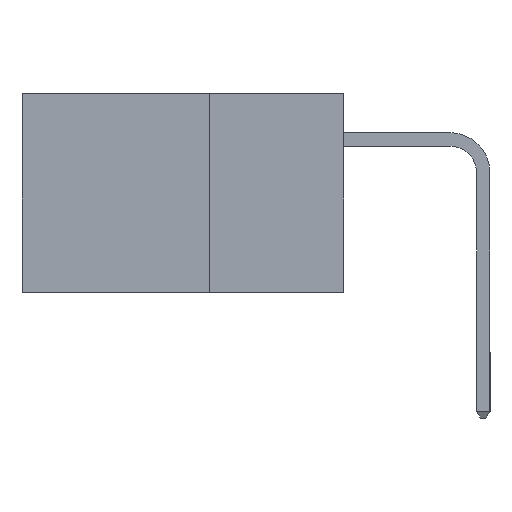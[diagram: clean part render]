
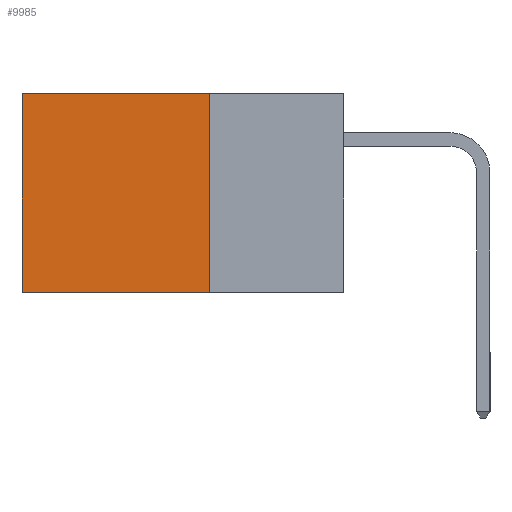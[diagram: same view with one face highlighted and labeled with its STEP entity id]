
A CAD part, left-side view. The second image highlights one B-rep face of the part: STEP entity #9985.
In plain terms, the highlighted planar face has unit normal (-1, 0, 0).
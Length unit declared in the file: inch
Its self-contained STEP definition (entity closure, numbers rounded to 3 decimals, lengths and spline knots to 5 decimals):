
#152 = CARTESIAN_POINT ( 'NONE',  ( 0.2615, 0.25, -0.37 ) ) ;
#375 = ORIENTED_EDGE ( 'NONE', *, *, #7150, .F. ) ;
#807 = LINE ( 'NONE', #12496, #3893 ) ;
#1291 = ORIENTED_EDGE ( 'NONE', *, *, #4926, .T. ) ;
#1694 = FACE_OUTER_BOUND ( 'NONE', #6108, .T. ) ;
#1975 = DIRECTION ( 'NONE',  ( 0., 1., 0. ) ) ;
#2666 = DIRECTION ( 'NONE',  ( 0., 0., -1. ) ) ;
#2728 = CARTESIAN_POINT ( 'NONE',  ( 0.2615, 0.25, -0.37 ) ) ;
#2804 = VERTEX_POINT ( 'NONE', #11179 ) ;
#2896 = DIRECTION ( 'NONE',  ( 0., 0., -1. ) ) ;
#3865 = DIRECTION ( 'NONE',  ( 1., 0., 0. ) ) ;
#3893 = VECTOR ( 'NONE', #10416, 39.37008 ) ;
#4850 = VECTOR ( 'NONE', #5221, 39.37008 ) ;
#4926 = EDGE_CURVE ( 'NONE', #12583, #6183, #807, .T. ) ;
#4931 = CARTESIAN_POINT ( 'NONE',  ( 0.2615, 0.25, -0.37 ) ) ;
#5221 = DIRECTION ( 'NONE',  ( 0., 0., -1. ) ) ;
#5616 = PLANE ( 'NONE',  #7283 ) ;
#6052 = ORIENTED_EDGE ( 'NONE', *, *, #8174, .T. ) ;
#6108 = EDGE_LOOP ( 'NONE', ( #6052, #375, #12393, #1291 ) ) ;
#6183 = VERTEX_POINT ( 'NONE', #7641 ) ;
#6530 = EDGE_CURVE ( 'NONE', #12583, #9135, #7627, .T. ) ;
#7150 = EDGE_CURVE ( 'NONE', #9135, #2804, #8033, .T. ) ;
#7283 = AXIS2_PLACEMENT_3D ( 'NONE', #8904, #3865, #2896 ) ;
#7627 = LINE ( 'NONE', #2728, #12087 ) ;
#7641 = CARTESIAN_POINT ( 'NONE',  ( 0.2615, 0.6, 0. ) ) ;
#8033 = LINE ( 'NONE', #4931, #11480 ) ;
#8174 = EDGE_CURVE ( 'NONE', #6183, #2804, #10319, .T. ) ;
#8623 = CARTESIAN_POINT ( 'NONE',  ( 0.2615, 0.25, 0. ) ) ;
#8904 = CARTESIAN_POINT ( 'NONE',  ( 0.2615, 0.25, -0.37 ) ) ;
#9135 = VERTEX_POINT ( 'NONE', #152 ) ;
#9233 = CARTESIAN_POINT ( 'NONE',  ( 0.2615, 0.6, -0.37 ) ) ;
#9985 = ADVANCED_FACE ( 'NONE', ( #1694 ), #5616, .F. ) ;
#10319 = LINE ( 'NONE', #9233, #4850 ) ;
#10416 = DIRECTION ( 'NONE',  ( 0., 1., 0. ) ) ;
#11179 = CARTESIAN_POINT ( 'NONE',  ( 0.2615, 0.6, -0.37 ) ) ;
#11480 = VECTOR ( 'NONE', #1975, 39.37008 ) ;
#12087 = VECTOR ( 'NONE', #2666, 39.37008 ) ;
#12393 = ORIENTED_EDGE ( 'NONE', *, *, #6530, .F. ) ;
#12496 = CARTESIAN_POINT ( 'NONE',  ( 0.2615, 0.25, 0. ) ) ;
#12583 = VERTEX_POINT ( 'NONE', #8623 ) ;
